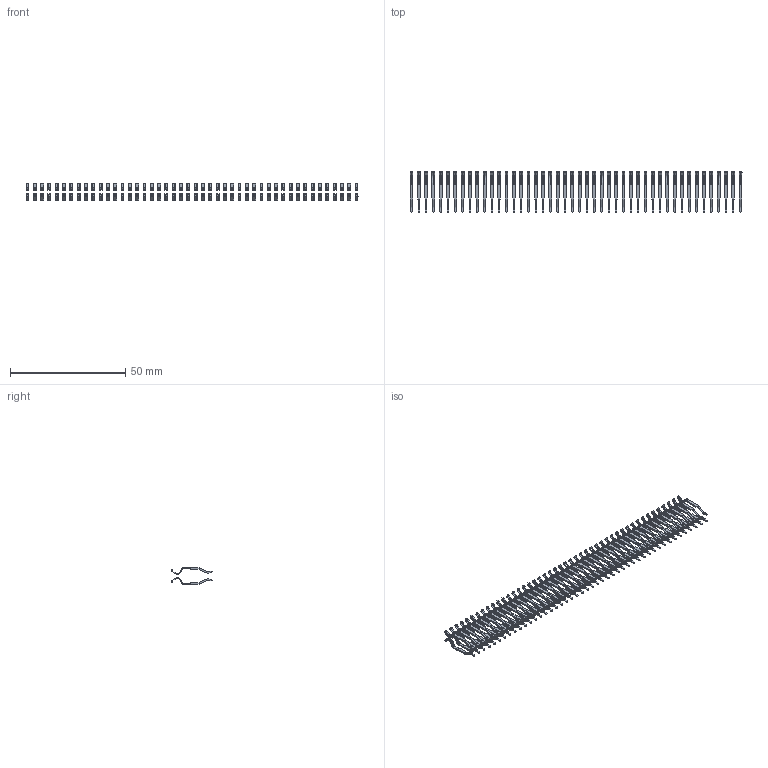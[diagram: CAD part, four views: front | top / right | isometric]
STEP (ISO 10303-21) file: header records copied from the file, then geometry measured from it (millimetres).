
FILE_DESCRIPTION (( 'STEP AP203' ), '1' );
FILE_NAME ('346-092-556-212.STEP', '2018-08-30T03:57:17', ( '' ), ( '' ), 'SwSTEP 2.0', 'SolidWorks 2016', '' );
FILE_SCHEMA (( 'CONFIG_CONTROL_DESIGN' ));
Length unit declared in the file: inch
Products named in the file (3): 346 Part_Flush Mounting Lugs - Side Mount; 345-292-001_556 Tail; 346-092-556-212
Assembly tree (93 placements, depth 2):
  346-092-556-212
    346 Part_Flush Mounting Lugs - Side Mount
    345-292-001_556 Tail  x92
Bounding box: 144.15 x 17.66 x 6.99 mm (x, y, z)
Volume: 824.2 mm3; surface area: 5821.9 mm2
Topology: 92 solids, 92 shells, 4784 faces, 13984 edges, 9200 vertices
Faces by surface type: plane 3128, cylinder 1656
Entity records: 29705 total; most frequent: CARTESIAN_POINT 4904, ORIENTED_EDGE 4826, DIRECTION 4361, EDGE_CURVE 2413, VECTOR 2089, LINE 2089, VERTEX_POINT 1606, AXIS2_PLACEMENT_3D 1136
